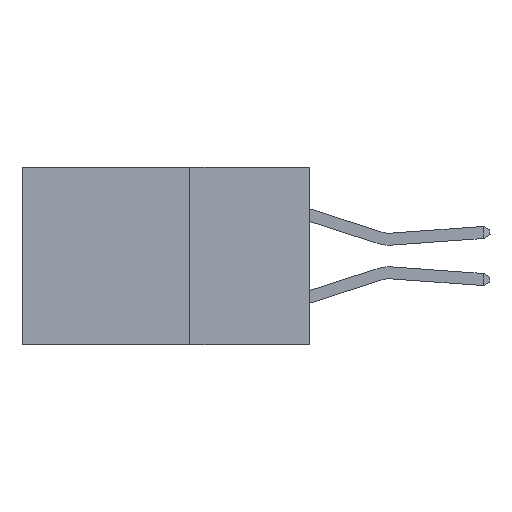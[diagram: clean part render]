
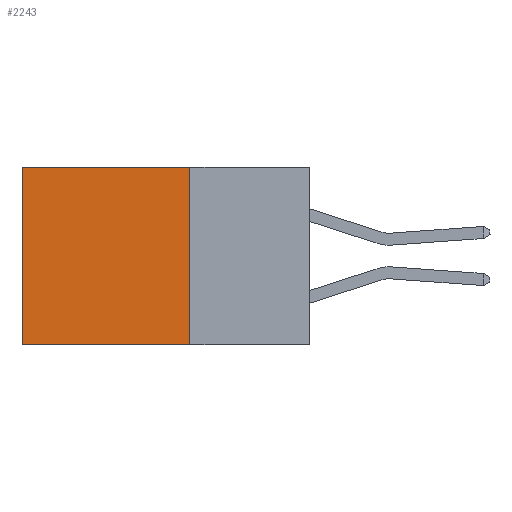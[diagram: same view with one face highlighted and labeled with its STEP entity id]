
A CAD part, left-side view. The second image highlights one B-rep face of the part: STEP entity #2243.
In plain terms, the highlighted planar face has unit normal (-1, 0, 0).
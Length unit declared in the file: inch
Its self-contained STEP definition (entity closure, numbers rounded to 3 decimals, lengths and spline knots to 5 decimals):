
#109 = EDGE_CURVE ( 'NONE', #7000, #9441, #1648, .T. ) ;
#349 = VECTOR ( 'NONE', #4941, 39.37008 ) ;
#956 = ORIENTED_EDGE ( 'NONE', *, *, #2579, .F. ) ;
#1050 = CARTESIAN_POINT ( 'NONE',  ( 0.2615, 0.25, 0. ) ) ;
#1648 = LINE ( 'NONE', #7030, #3346 ) ;
#2146 = CARTESIAN_POINT ( 'NONE',  ( 0.2615, 0.25, -0.37 ) ) ;
#2243 = ADVANCED_FACE ( 'NONE', ( #3597 ), #5289, .F. ) ;
#2403 = VERTEX_POINT ( 'NONE', #3580 ) ;
#2579 = EDGE_CURVE ( 'NONE', #5166, #7000, #5424, .T. ) ;
#3112 = VECTOR ( 'NONE', #10226, 39.37008 ) ;
#3121 = CARTESIAN_POINT ( 'NONE',  ( 0.2615, 0.6, -0.37 ) ) ;
#3346 = VECTOR ( 'NONE', #5631, 39.37008 ) ;
#3580 = CARTESIAN_POINT ( 'NONE',  ( 0.2615, 0.6, 0. ) ) ;
#3597 = FACE_OUTER_BOUND ( 'NONE', #5596, .T. ) ;
#3639 = ORIENTED_EDGE ( 'NONE', *, *, #109, .F. ) ;
#3788 = VECTOR ( 'NONE', #6319, 39.37008 ) ;
#3898 = LINE ( 'NONE', #3121, #3788 ) ;
#4005 = EDGE_CURVE ( 'NONE', #2403, #9441, #3898, .T. ) ;
#4701 = CARTESIAN_POINT ( 'NONE',  ( 0.2615, 0.25, 0. ) ) ;
#4918 = CARTESIAN_POINT ( 'NONE',  ( 0.2615, 0.25, -0.37 ) ) ;
#4941 = DIRECTION ( 'NONE',  ( 0., 1., 0. ) ) ;
#5166 = VERTEX_POINT ( 'NONE', #4701 ) ;
#5289 = PLANE ( 'NONE',  #8943 ) ;
#5424 = LINE ( 'NONE', #8602, #3112 ) ;
#5596 = EDGE_LOOP ( 'NONE', ( #7234, #3639, #956, #7151 ) ) ;
#5631 = DIRECTION ( 'NONE',  ( 0., 1., 0. ) ) ;
#6319 = DIRECTION ( 'NONE',  ( 0., 0., -1. ) ) ;
#6746 = CARTESIAN_POINT ( 'NONE',  ( 0.2615, 0.6, -0.37 ) ) ;
#6791 = DIRECTION ( 'NONE',  ( 0., 0., -1. ) ) ;
#6846 = DIRECTION ( 'NONE',  ( 1., 0., 0. ) ) ;
#7000 = VERTEX_POINT ( 'NONE', #4918 ) ;
#7030 = CARTESIAN_POINT ( 'NONE',  ( 0.2615, 0.25, -0.37 ) ) ;
#7151 = ORIENTED_EDGE ( 'NONE', *, *, #9269, .T. ) ;
#7231 = LINE ( 'NONE', #1050, #349 ) ;
#7234 = ORIENTED_EDGE ( 'NONE', *, *, #4005, .T. ) ;
#8602 = CARTESIAN_POINT ( 'NONE',  ( 0.2615, 0.25, -0.37 ) ) ;
#8943 = AXIS2_PLACEMENT_3D ( 'NONE', #2146, #6846, #6791 ) ;
#9269 = EDGE_CURVE ( 'NONE', #5166, #2403, #7231, .T. ) ;
#9441 = VERTEX_POINT ( 'NONE', #6746 ) ;
#10226 = DIRECTION ( 'NONE',  ( 0., 0., -1. ) ) ;
